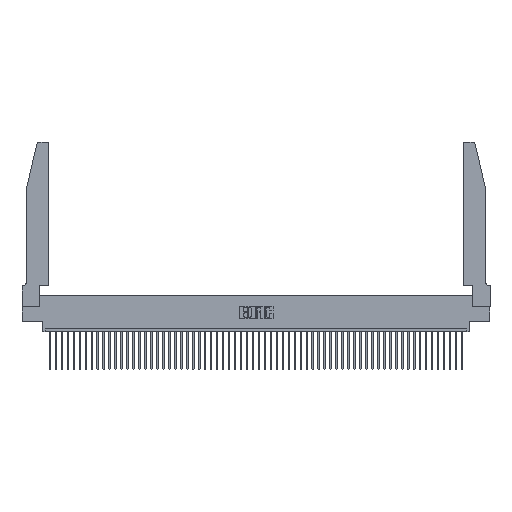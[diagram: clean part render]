
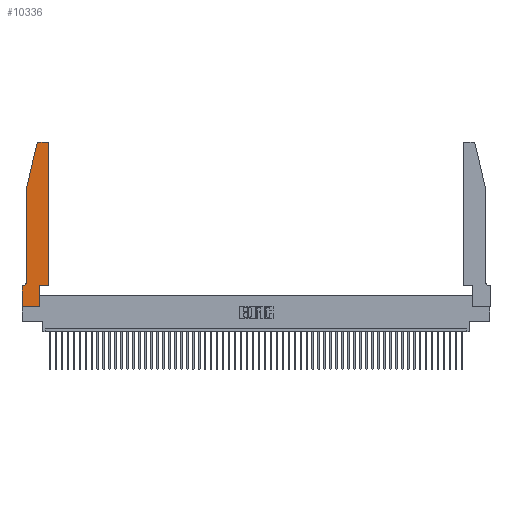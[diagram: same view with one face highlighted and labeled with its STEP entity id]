
A CAD part, top view. The second image highlights one B-rep face of the part: STEP entity #10336.
In plain terms, the highlighted planar face has unit normal (0, 0, 1).
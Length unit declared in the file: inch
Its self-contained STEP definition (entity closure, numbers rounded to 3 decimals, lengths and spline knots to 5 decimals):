
#577 = CARTESIAN_POINT ( 'NONE',  ( 0.4505, 0.35, 0.37 ) ) ;
#756 = DIRECTION ( 'NONE',  ( 0., 0., -1. ) ) ;
#855 = EDGE_CURVE ( 'NONE', #18200, #19691, #51378, .T. ) ;
#1281 = VECTOR ( 'NONE', #52190, 39.37008 ) ;
#2510 = ORIENTED_EDGE ( 'NONE', *, *, #25898, .T. ) ;
#3728 = ORIENTED_EDGE ( 'NONE', *, *, #44359, .T. ) ;
#4904 = DIRECTION ( 'NONE',  ( 1., 0., 0. ) ) ;
#5385 = ORIENTED_EDGE ( 'NONE', *, *, #855, .T. ) ;
#5442 = PLANE ( 'NONE',  #8613 ) ;
#5448 = CARTESIAN_POINT ( 'NONE',  ( 0.0055, 0.42, 0.37 ) ) ;
#7476 = DIRECTION ( 'NONE',  ( 0., 0., 1. ) ) ;
#7624 = DIRECTION ( 'NONE',  ( 0., 0., 1. ) ) ;
#8613 = AXIS2_PLACEMENT_3D ( 'NONE', #18588, #49714, #40848 ) ;
#9999 = DIRECTION ( 'NONE',  ( -0.239, -0.971, 0. ) ) ;
#10336 = ADVANCED_FACE ( 'NONE', ( #39385 ), #5442, .T. ) ;
#10787 = CARTESIAN_POINT ( 'NONE',  ( 0., 0., 0.37 ) ) ;
#11108 = DIRECTION ( 'NONE',  ( 0., -1., 0. ) ) ;
#11548 = VERTEX_POINT ( 'NONE', #37431 ) ;
#11612 = DIRECTION ( 'NONE',  ( 1., 0., 0. ) ) ;
#11746 = CARTESIAN_POINT ( 'NONE',  ( 0.2605, 2.75, 0.37 ) ) ;
#11918 = LINE ( 'NONE', #11746, #31497 ) ;
#13225 = DIRECTION ( 'NONE',  ( -1., 0., 0. ) ) ;
#13588 = EDGE_CURVE ( 'NONE', #25046, #25578, #50039, .T. ) ;
#14353 = LINE ( 'NONE', #23379, #37115 ) ;
#14599 = ORIENTED_EDGE ( 'NONE', *, *, #48237, .T. ) ;
#14686 = CARTESIAN_POINT ( 'NONE',  ( 0.284, 2.72, 0.37 ) ) ;
#14952 = VERTEX_POINT ( 'NONE', #28503 ) ;
#15518 = CARTESIAN_POINT ( 'NONE',  ( 0.0755, 0.42, 0.37 ) ) ;
#17293 = ORIENTED_EDGE ( 'NONE', *, *, #13588, .T. ) ;
#17473 = AXIS2_PLACEMENT_3D ( 'NONE', #14686, #7624, #23101 ) ;
#17547 = VECTOR ( 'NONE', #25518, 39.37008 ) ;
#17912 = VECTOR ( 'NONE', #4904, 39.37008 ) ;
#18200 = VERTEX_POINT ( 'NONE', #18992 ) ;
#18588 = CARTESIAN_POINT ( 'NONE',  ( 0., 0.35, 0.37 ) ) ;
#18801 = VECTOR ( 'NONE', #22845, 39.37008 ) ;
#18806 = LINE ( 'NONE', #577, #17912 ) ;
#18992 = CARTESIAN_POINT ( 'NONE',  ( 0.0055, 0.35, 0.37 ) ) ;
#19478 = AXIS2_PLACEMENT_3D ( 'NONE', #5448, #756, #13225 ) ;
#19691 = VERTEX_POINT ( 'NONE', #53272 ) ;
#19762 = VERTEX_POINT ( 'NONE', #15518 ) ;
#20115 = EDGE_CURVE ( 'NONE', #25578, #22437, #30463, .T. ) ;
#20598 = DIRECTION ( 'NONE',  ( -1., 0., 0. ) ) ;
#21843 = ORIENTED_EDGE ( 'NONE', *, *, #50194, .T. ) ;
#22409 = EDGE_CURVE ( 'NONE', #43604, #40335, #31977, .T. ) ;
#22437 = VERTEX_POINT ( 'NONE', #49676 ) ;
#22625 = ORIENTED_EDGE ( 'NONE', *, *, #48524, .T. ) ;
#22845 = DIRECTION ( 'NONE',  ( 0., -1., 0. ) ) ;
#23101 = DIRECTION ( 'NONE',  ( 1., 0., 0. ) ) ;
#23117 = CARTESIAN_POINT ( 'NONE',  ( 0.4505, 0.35, 0.37 ) ) ;
#23379 = CARTESIAN_POINT ( 'NONE',  ( 0.0755, 2., 0.37 ) ) ;
#23575 = CARTESIAN_POINT ( 'NONE',  ( 0.0755, 2., 0.37 ) ) ;
#23723 = CARTESIAN_POINT ( 'NONE',  ( 0.4205, 2.72, 0.37 ) ) ;
#23929 = EDGE_CURVE ( 'NONE', #40335, #25046, #18806, .T. ) ;
#24577 = VERTEX_POINT ( 'NONE', #24734 ) ;
#24734 = CARTESIAN_POINT ( 'NONE',  ( 0.0755, 2., 0.37 ) ) ;
#25046 = VERTEX_POINT ( 'NONE', #42690 ) ;
#25518 = DIRECTION ( 'NONE',  ( 1., 0., 0. ) ) ;
#25578 = VERTEX_POINT ( 'NONE', #39368 ) ;
#25898 = EDGE_CURVE ( 'NONE', #28225, #11548, #53649, .T. ) ;
#26475 = EDGE_CURVE ( 'NONE', #22437, #28225, #11918, .T. ) ;
#27411 = ORIENTED_EDGE ( 'NONE', *, *, #26475, .T. ) ;
#27705 = EDGE_CURVE ( 'NONE', #14952, #43604, #50092, .T. ) ;
#28137 = ORIENTED_EDGE ( 'NONE', *, *, #20115, .T. ) ;
#28225 = VERTEX_POINT ( 'NONE', #39583 ) ;
#28503 = CARTESIAN_POINT ( 'NONE',  ( 0., 0., 0.37 ) ) ;
#28706 = VECTOR ( 'NONE', #20598, 39.37008 ) ;
#28861 = LINE ( 'NONE', #23575, #36668 ) ;
#30463 = CIRCLE ( 'NONE', #50022, 0.03 ) ;
#30777 = ORIENTED_EDGE ( 'NONE', *, *, #22409, .T. ) ;
#31497 = VECTOR ( 'NONE', #36874, 39.37008 ) ;
#31977 = LINE ( 'NONE', #53069, #37124 ) ;
#32711 = CIRCLE ( 'NONE', #19478, 0.07 ) ;
#36668 = VECTOR ( 'NONE', #9999, 39.37008 ) ;
#36874 = DIRECTION ( 'NONE',  ( -1., 0., 0. ) ) ;
#37115 = VECTOR ( 'NONE', #11108, 39.37008 ) ;
#37124 = VECTOR ( 'NONE', #37191, 39.37008 ) ;
#37191 = DIRECTION ( 'NONE',  ( 0., 1., 0. ) ) ;
#37409 = CARTESIAN_POINT ( 'NONE',  ( 0.2865, 0., 0.37 ) ) ;
#37431 = CARTESIAN_POINT ( 'NONE',  ( 0.25487, 2.72718, 0.37 ) ) ;
#37680 = CARTESIAN_POINT ( 'NONE',  ( 0., 0., 0.37 ) ) ;
#39368 = CARTESIAN_POINT ( 'NONE',  ( 0.4505, 2.72, 0.37 ) ) ;
#39385 = FACE_OUTER_BOUND ( 'NONE', #45869, .T. ) ;
#39583 = CARTESIAN_POINT ( 'NONE',  ( 0.284, 2.75, 0.37 ) ) ;
#40335 = VERTEX_POINT ( 'NONE', #49744 ) ;
#40848 = DIRECTION ( 'NONE',  ( 1., 0., 0. ) ) ;
#40914 = LINE ( 'NONE', #10787, #18801 ) ;
#42690 = CARTESIAN_POINT ( 'NONE',  ( 0.4505, 0.35, 0.37 ) ) ;
#42699 = ORIENTED_EDGE ( 'NONE', *, *, #23929, .T. ) ;
#43604 = VERTEX_POINT ( 'NONE', #37409 ) ;
#44359 = EDGE_CURVE ( 'NONE', #19691, #14952, #40914, .T. ) ;
#45118 = CARTESIAN_POINT ( 'NONE',  ( 0.0755, 0.35, 0.37 ) ) ;
#45869 = EDGE_LOOP ( 'NONE', ( #27411, #2510, #14599, #21843, #22625, #5385, #3728, #53131, #30777, #42699, #17293, #28137 ) ) ;
#48237 = EDGE_CURVE ( 'NONE', #11548, #24577, #28861, .T. ) ;
#48524 = EDGE_CURVE ( 'NONE', #19762, #18200, #32711, .T. ) ;
#49676 = CARTESIAN_POINT ( 'NONE',  ( 0.4205, 2.75, 0.37 ) ) ;
#49714 = DIRECTION ( 'NONE',  ( 0., 0., 1. ) ) ;
#49744 = CARTESIAN_POINT ( 'NONE',  ( 0.2865, 0.35, 0.37 ) ) ;
#50022 = AXIS2_PLACEMENT_3D ( 'NONE', #23723, #7476, #11612 ) ;
#50039 = LINE ( 'NONE', #23117, #1281 ) ;
#50092 = LINE ( 'NONE', #37680, #17547 ) ;
#50194 = EDGE_CURVE ( 'NONE', #24577, #19762, #14353, .T. ) ;
#51378 = LINE ( 'NONE', #45118, #28706 ) ;
#52190 = DIRECTION ( 'NONE',  ( 0., 1., 0. ) ) ;
#53069 = CARTESIAN_POINT ( 'NONE',  ( 0.2865, 0.35, 0.37 ) ) ;
#53131 = ORIENTED_EDGE ( 'NONE', *, *, #27705, .T. ) ;
#53272 = CARTESIAN_POINT ( 'NONE',  ( 0., 0.35, 0.37 ) ) ;
#53649 = CIRCLE ( 'NONE', #17473, 0.03 ) ;
